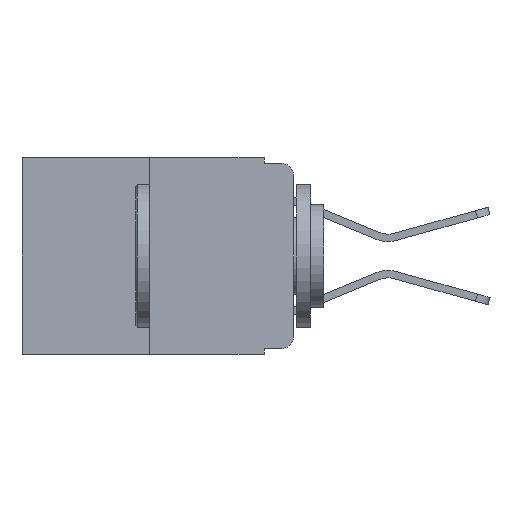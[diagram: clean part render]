
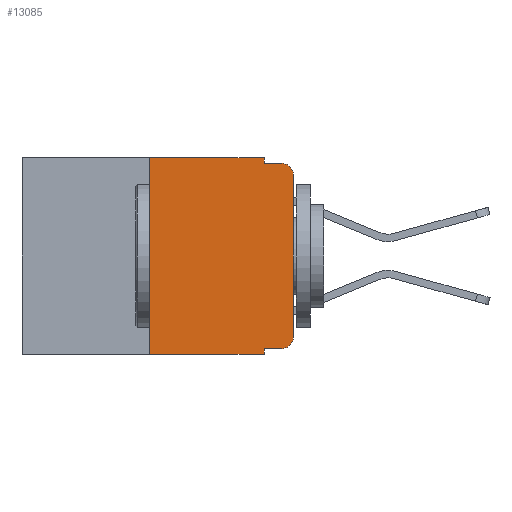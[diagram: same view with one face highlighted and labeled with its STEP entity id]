
A CAD part, left-side view. The second image highlights one B-rep face of the part: STEP entity #13085.
In plain terms, the highlighted planar face has unit normal (-1, 0, 0).
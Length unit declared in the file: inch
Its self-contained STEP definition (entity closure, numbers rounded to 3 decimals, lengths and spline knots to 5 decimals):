
#65 = VERTEX_POINT ( 'NONE', #17495 ) ;
#178 = EDGE_CURVE ( 'NONE', #8128, #17938, #10564, .T. ) ;
#437 = CARTESIAN_POINT ( 'NONE',  ( 0., 0.051, 0. ) ) ;
#529 = ORIENTED_EDGE ( 'NONE', *, *, #19183, .F. ) ;
#996 = VECTOR ( 'NONE', #17705, 39.37008 ) ;
#998 = ORIENTED_EDGE ( 'NONE', *, *, #178, .F. ) ;
#1143 = ORIENTED_EDGE ( 'NONE', *, *, #11216, .F. ) ;
#1802 = VERTEX_POINT ( 'NONE', #19628 ) ;
#1861 = DIRECTION ( 'NONE',  ( 0., 0., -1. ) ) ;
#2048 = EDGE_CURVE ( 'NONE', #6310, #13308, #21632, .T. ) ;
#2325 = VERTEX_POINT ( 'NONE', #17932 ) ;
#2604 = EDGE_LOOP ( 'NONE', ( #3569, #6663, #998, #15568, #1143, #4011, #18336, #529, #18790, #17251 ) ) ;
#2830 = CIRCLE ( 'NONE', #16426, 0.02 ) ;
#3569 = ORIENTED_EDGE ( 'NONE', *, *, #12727, .T. ) ;
#3743 = CARTESIAN_POINT ( 'NONE',  ( 0., 0.051, -0.343 ) ) ;
#3754 = DIRECTION ( 'NONE',  ( 0., 0., -1. ) ) ;
#4011 = ORIENTED_EDGE ( 'NONE', *, *, #2048, .F. ) ;
#4267 = DIRECTION ( 'NONE',  ( -1., 0., 0. ) ) ;
#4827 = VECTOR ( 'NONE', #22239, 39.37008 ) ;
#4854 = LINE ( 'NONE', #6027, #18966 ) ;
#5384 = VECTOR ( 'NONE', #19389, 39.37008 ) ;
#6027 = CARTESIAN_POINT ( 'NONE',  ( 0., 0.473, 0. ) ) ;
#6310 = VERTEX_POINT ( 'NONE', #12341 ) ;
#6634 = CARTESIAN_POINT ( 'NONE',  ( 0., 0.02, -0.01 ) ) ;
#6663 = ORIENTED_EDGE ( 'NONE', *, *, #9702, .T. ) ;
#6748 = EDGE_CURVE ( 'NONE', #8642, #65, #17978, .T. ) ;
#7170 = DIRECTION ( 'NONE',  ( -1., 0., 0. ) ) ;
#7870 = VECTOR ( 'NONE', #12304, 39.37008 ) ;
#8128 = VERTEX_POINT ( 'NONE', #13522 ) ;
#8286 = CARTESIAN_POINT ( 'NONE',  ( 0., 0.473, 0. ) ) ;
#8303 = CARTESIAN_POINT ( 'NONE',  ( 0., 0.473, -0.343 ) ) ;
#8309 = CARTESIAN_POINT ( 'NONE',  ( 0., 0.25, 0. ) ) ;
#8642 = VERTEX_POINT ( 'NONE', #15428 ) ;
#8968 = CARTESIAN_POINT ( 'NONE',  ( 0., 0.02, -0.313 ) ) ;
#9492 = CARTESIAN_POINT ( 'NONE',  ( 0., 0.051, -0.333 ) ) ;
#9518 = LINE ( 'NONE', #12499, #14373 ) ;
#9675 = DIRECTION ( 'NONE',  ( 0., -1., 0. ) ) ;
#9702 = EDGE_CURVE ( 'NONE', #2325, #17938, #12596, .T. ) ;
#9707 = LINE ( 'NONE', #437, #5384 ) ;
#10122 = VECTOR ( 'NONE', #18927, 39.37008 ) ;
#10564 = LINE ( 'NONE', #17863, #7870 ) ;
#11216 = EDGE_CURVE ( 'NONE', #13308, #1802, #4854, .T. ) ;
#12011 = LINE ( 'NONE', #8303, #10122 ) ;
#12304 = DIRECTION ( 'NONE',  ( 0., -1., 0. ) ) ;
#12341 = CARTESIAN_POINT ( 'NONE',  ( 0., 0.25, -0.343 ) ) ;
#12499 = CARTESIAN_POINT ( 'NONE',  ( 0., 0.051, 0. ) ) ;
#12596 = CIRCLE ( 'NONE', #15963, 0.02 ) ;
#12727 = EDGE_CURVE ( 'NONE', #16703, #2325, #22403, .T. ) ;
#13085 = ADVANCED_FACE ( 'NONE', ( #15340 ), #13626, .F. ) ;
#13308 = VERTEX_POINT ( 'NONE', #15985 ) ;
#13522 = CARTESIAN_POINT ( 'NONE',  ( 0., 0.051, -0.01 ) ) ;
#13626 = PLANE ( 'NONE',  #13968 ) ;
#13968 = AXIS2_PLACEMENT_3D ( 'NONE', #8286, #15238, #21984 ) ;
#14105 = CARTESIAN_POINT ( 'NONE',  ( 0., 0., 0. ) ) ;
#14373 = VECTOR ( 'NONE', #3754, 39.37008 ) ;
#14375 = EDGE_CURVE ( 'NONE', #6310, #16860, #12011, .T. ) ;
#15238 = DIRECTION ( 'NONE',  ( 1., 0., 0. ) ) ;
#15340 = FACE_OUTER_BOUND ( 'NONE', #2604, .T. ) ;
#15428 = CARTESIAN_POINT ( 'NONE',  ( 0., 0.051, -0.333 ) ) ;
#15568 = ORIENTED_EDGE ( 'NONE', *, *, #20421, .F. ) ;
#15963 = AXIS2_PLACEMENT_3D ( 'NONE', #20096, #4267, #18425 ) ;
#15985 = CARTESIAN_POINT ( 'NONE',  ( 0., 0.25, 0. ) ) ;
#16303 = DIRECTION ( 'NONE',  ( 0., -1., 0. ) ) ;
#16426 = AXIS2_PLACEMENT_3D ( 'NONE', #8968, #7170, #1861 ) ;
#16703 = VERTEX_POINT ( 'NONE', #18834 ) ;
#16860 = VERTEX_POINT ( 'NONE', #3743 ) ;
#17251 = ORIENTED_EDGE ( 'NONE', *, *, #22343, .T. ) ;
#17495 = CARTESIAN_POINT ( 'NONE',  ( 0., 0.02, -0.333 ) ) ;
#17705 = DIRECTION ( 'NONE',  ( 0., 0., 1. ) ) ;
#17863 = CARTESIAN_POINT ( 'NONE',  ( 0., 0.051, -0.01 ) ) ;
#17932 = CARTESIAN_POINT ( 'NONE',  ( 0., 0., -0.03 ) ) ;
#17938 = VERTEX_POINT ( 'NONE', #6634 ) ;
#17978 = LINE ( 'NONE', #9492, #21246 ) ;
#18336 = ORIENTED_EDGE ( 'NONE', *, *, #14375, .T. ) ;
#18425 = DIRECTION ( 'NONE',  ( 0., 0., -1. ) ) ;
#18790 = ORIENTED_EDGE ( 'NONE', *, *, #6748, .T. ) ;
#18834 = CARTESIAN_POINT ( 'NONE',  ( 0., 0., -0.313 ) ) ;
#18927 = DIRECTION ( 'NONE',  ( 0., -1., 0. ) ) ;
#18966 = VECTOR ( 'NONE', #9675, 39.37008 ) ;
#19183 = EDGE_CURVE ( 'NONE', #8642, #16860, #9518, .T. ) ;
#19389 = DIRECTION ( 'NONE',  ( 0., 0., -1. ) ) ;
#19628 = CARTESIAN_POINT ( 'NONE',  ( 0., 0.051, 0. ) ) ;
#20096 = CARTESIAN_POINT ( 'NONE',  ( 0., 0.02, -0.03 ) ) ;
#20421 = EDGE_CURVE ( 'NONE', #1802, #8128, #9707, .T. ) ;
#21246 = VECTOR ( 'NONE', #16303, 39.37008 ) ;
#21632 = LINE ( 'NONE', #8309, #4827 ) ;
#21984 = DIRECTION ( 'NONE',  ( 0., 0., -1. ) ) ;
#22239 = DIRECTION ( 'NONE',  ( 0., 0., 1. ) ) ;
#22343 = EDGE_CURVE ( 'NONE', #65, #16703, #2830, .T. ) ;
#22403 = LINE ( 'NONE', #14105, #996 ) ;
